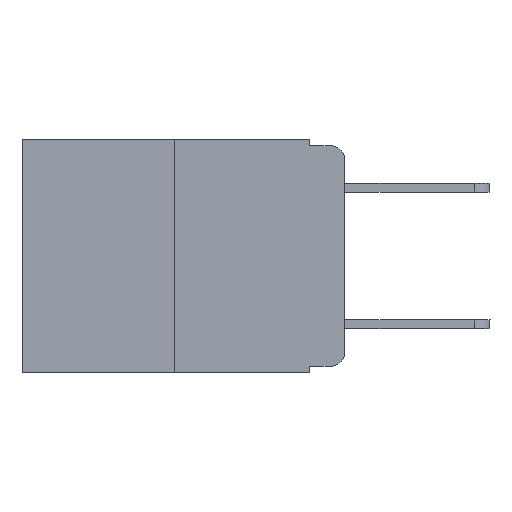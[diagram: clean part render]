
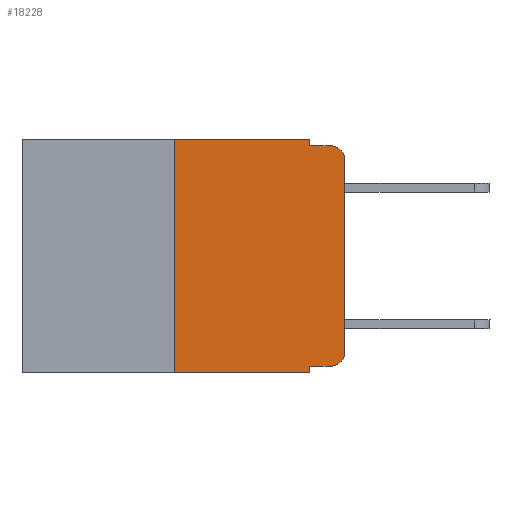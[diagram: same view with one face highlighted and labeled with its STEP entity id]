
A CAD part, left-side view. The second image highlights one B-rep face of the part: STEP entity #18228.
In plain terms, the highlighted planar face has unit normal (-1, 0, 0).
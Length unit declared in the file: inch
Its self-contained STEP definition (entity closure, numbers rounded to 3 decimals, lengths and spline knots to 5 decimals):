
#96 = EDGE_CURVE ( 'NONE', #23106, #5481, #2008, .T. ) ;
#411 = LINE ( 'NONE', #15471, #7386 ) ;
#634 = DIRECTION ( 'NONE',  ( 0., 0., -1. ) ) ;
#685 = VECTOR ( 'NONE', #13310, 39.37008 ) ;
#1140 = VECTOR ( 'NONE', #16153, 39.37008 ) ;
#2008 = LINE ( 'NONE', #5016, #1140 ) ;
#2118 = EDGE_CURVE ( 'NONE', #3535, #12338, #11757, .T. ) ;
#2185 = CARTESIAN_POINT ( 'NONE',  ( 0., 0.051, 0. ) ) ;
#2246 = CARTESIAN_POINT ( 'NONE',  ( 0., 0.051, -0.333 ) ) ;
#2453 = CARTESIAN_POINT ( 'NONE',  ( 0., 0.051, -0.01 ) ) ;
#2509 = ORIENTED_EDGE ( 'NONE', *, *, #5224, .F. ) ;
#2716 = ORIENTED_EDGE ( 'NONE', *, *, #22798, .T. ) ;
#2856 = CARTESIAN_POINT ( 'NONE',  ( 0., 0.25, -0.343 ) ) ;
#2903 = DIRECTION ( 'NONE',  ( 1., 0., 0. ) ) ;
#2927 = DIRECTION ( 'NONE',  ( 0., -1., 0. ) ) ;
#3284 = LINE ( 'NONE', #15128, #5037 ) ;
#3535 = VERTEX_POINT ( 'NONE', #12532 ) ;
#3777 = CARTESIAN_POINT ( 'NONE',  ( 0., 0., -0.03 ) ) ;
#5016 = CARTESIAN_POINT ( 'NONE',  ( 0., 0.473, -0.343 ) ) ;
#5037 = VECTOR ( 'NONE', #7702, 39.37008 ) ;
#5224 = EDGE_CURVE ( 'NONE', #17635, #10416, #20629, .T. ) ;
#5481 = VERTEX_POINT ( 'NONE', #17708 ) ;
#5524 = ORIENTED_EDGE ( 'NONE', *, *, #2118, .T. ) ;
#5618 = CARTESIAN_POINT ( 'NONE',  ( 0., 0.051, -0.01 ) ) ;
#5712 = AXIS2_PLACEMENT_3D ( 'NONE', #20546, #14894, #9582 ) ;
#5952 = AXIS2_PLACEMENT_3D ( 'NONE', #23014, #2903, #23503 ) ;
#6067 = CARTESIAN_POINT ( 'NONE',  ( 0., 0.02, -0.03 ) ) ;
#7307 = ORIENTED_EDGE ( 'NONE', *, *, #16744, .F. ) ;
#7386 = VECTOR ( 'NONE', #8059, 39.37008 ) ;
#7599 = AXIS2_PLACEMENT_3D ( 'NONE', #6067, #9553, #16992 ) ;
#7659 = ORIENTED_EDGE ( 'NONE', *, *, #96, .T. ) ;
#7702 = DIRECTION ( 'NONE',  ( 0., 0., 1. ) ) ;
#7946 = CARTESIAN_POINT ( 'NONE',  ( 0., 0., 0. ) ) ;
#8059 = DIRECTION ( 'NONE',  ( 0., -1., 0. ) ) ;
#8596 = ORIENTED_EDGE ( 'NONE', *, *, #23522, .T. ) ;
#8738 = LINE ( 'NONE', #2185, #16532 ) ;
#8743 = ORIENTED_EDGE ( 'NONE', *, *, #10969, .F. ) ;
#9553 = DIRECTION ( 'NONE',  ( -1., 0., 0. ) ) ;
#9582 = DIRECTION ( 'NONE',  ( 0., 0., -1. ) ) ;
#9995 = CIRCLE ( 'NONE', #5712, 0.02 ) ;
#10099 = PLANE ( 'NONE',  #5952 ) ;
#10174 = CIRCLE ( 'NONE', #7599, 0.02 ) ;
#10199 = CARTESIAN_POINT ( 'NONE',  ( 0., 0.051, -0.333 ) ) ;
#10416 = VERTEX_POINT ( 'NONE', #2453 ) ;
#10969 = EDGE_CURVE ( 'NONE', #23106, #22913, #3284, .T. ) ;
#11077 = FACE_OUTER_BOUND ( 'NONE', #20507, .T. ) ;
#11542 = CARTESIAN_POINT ( 'NONE',  ( 0., 0.051, 0. ) ) ;
#11735 = DIRECTION ( 'NONE',  ( 0., 0., 1. ) ) ;
#11757 = LINE ( 'NONE', #7946, #15801 ) ;
#12338 = VERTEX_POINT ( 'NONE', #3777 ) ;
#12532 = CARTESIAN_POINT ( 'NONE',  ( 0., 0., -0.313 ) ) ;
#13045 = LINE ( 'NONE', #10199, #19424 ) ;
#13094 = VERTEX_POINT ( 'NONE', #19047 ) ;
#13310 = DIRECTION ( 'NONE',  ( 0., 0., -1. ) ) ;
#13586 = ORIENTED_EDGE ( 'NONE', *, *, #18777, .T. ) ;
#13628 = EDGE_CURVE ( 'NONE', #10416, #20417, #19651, .T. ) ;
#14829 = ORIENTED_EDGE ( 'NONE', *, *, #18741, .F. ) ;
#14894 = DIRECTION ( 'NONE',  ( -1., 0., 0. ) ) ;
#15128 = CARTESIAN_POINT ( 'NONE',  ( 0., 0.25, 0. ) ) ;
#15452 = CARTESIAN_POINT ( 'NONE',  ( 0., 0.25, 0. ) ) ;
#15471 = CARTESIAN_POINT ( 'NONE',  ( 0., 0.473, 0. ) ) ;
#15801 = VECTOR ( 'NONE', #11735, 39.37008 ) ;
#16153 = DIRECTION ( 'NONE',  ( 0., -1., 0. ) ) ;
#16484 = VECTOR ( 'NONE', #18561, 39.37008 ) ;
#16532 = VECTOR ( 'NONE', #634, 39.37008 ) ;
#16744 = EDGE_CURVE ( 'NONE', #22913, #17635, #411, .T. ) ;
#16992 = DIRECTION ( 'NONE',  ( 0., 0., -1. ) ) ;
#17635 = VERTEX_POINT ( 'NONE', #23450 ) ;
#17708 = CARTESIAN_POINT ( 'NONE',  ( 0., 0.051, -0.343 ) ) ;
#18228 = ADVANCED_FACE ( 'NONE', ( #11077 ), #10099, .F. ) ;
#18561 = DIRECTION ( 'NONE',  ( 0., -1., 0. ) ) ;
#18741 = EDGE_CURVE ( 'NONE', #21099, #5481, #8738, .T. ) ;
#18777 = EDGE_CURVE ( 'NONE', #21099, #13094, #13045, .T. ) ;
#19047 = CARTESIAN_POINT ( 'NONE',  ( 0., 0.02, -0.333 ) ) ;
#19081 = ORIENTED_EDGE ( 'NONE', *, *, #13628, .F. ) ;
#19424 = VECTOR ( 'NONE', #2927, 39.37008 ) ;
#19651 = LINE ( 'NONE', #5618, #16484 ) ;
#20417 = VERTEX_POINT ( 'NONE', #22230 ) ;
#20507 = EDGE_LOOP ( 'NONE', ( #5524, #8596, #19081, #2509, #7307, #8743, #7659, #14829, #13586, #2716 ) ) ;
#20546 = CARTESIAN_POINT ( 'NONE',  ( 0., 0.02, -0.313 ) ) ;
#20629 = LINE ( 'NONE', #11542, #685 ) ;
#21099 = VERTEX_POINT ( 'NONE', #2246 ) ;
#22230 = CARTESIAN_POINT ( 'NONE',  ( 0., 0.02, -0.01 ) ) ;
#22798 = EDGE_CURVE ( 'NONE', #13094, #3535, #9995, .T. ) ;
#22913 = VERTEX_POINT ( 'NONE', #15452 ) ;
#23014 = CARTESIAN_POINT ( 'NONE',  ( 0., 0.473, 0. ) ) ;
#23106 = VERTEX_POINT ( 'NONE', #2856 ) ;
#23450 = CARTESIAN_POINT ( 'NONE',  ( 0., 0.051, 0. ) ) ;
#23503 = DIRECTION ( 'NONE',  ( 0., 0., -1. ) ) ;
#23522 = EDGE_CURVE ( 'NONE', #12338, #20417, #10174, .T. ) ;
